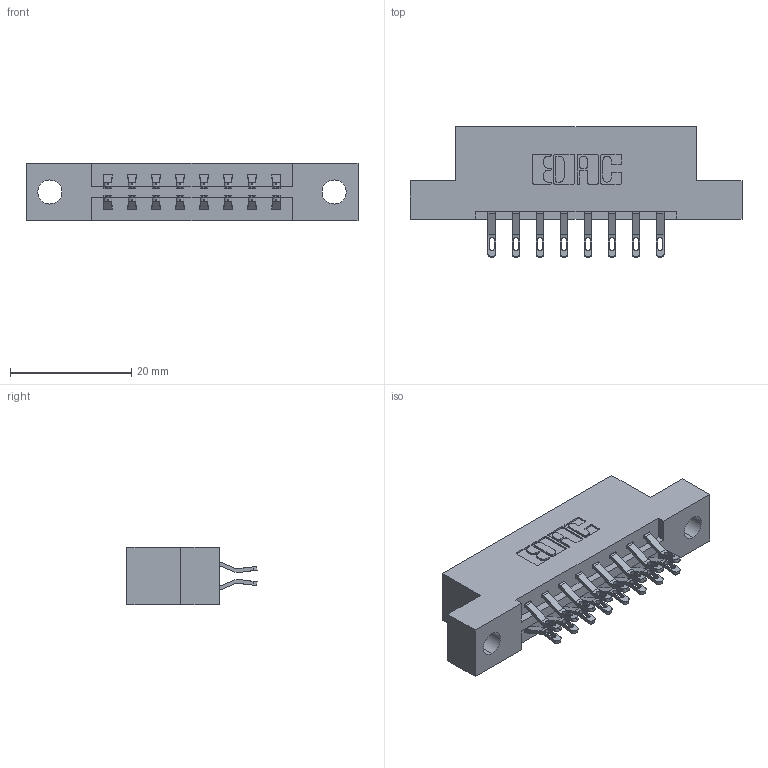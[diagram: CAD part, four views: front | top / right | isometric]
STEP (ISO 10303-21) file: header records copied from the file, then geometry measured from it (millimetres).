
FILE_DESCRIPTION (( 'STEP AP203' ), '1' );
FILE_NAME ('387-016-555-204.STEP', '2018-09-11T11:51:44', ( '' ), ( '' ), 'SwSTEP 2.0', 'SolidWorks 2016', '' );
FILE_SCHEMA (( 'CONFIG_CONTROL_DESIGN' ));
Length unit declared in the file: inch
Products named in the file (3): 387-016-555-204; 337 Part_Flush Mounting Lugs - 0.156 Dia-TH; 345-292-001_555 Tail
Assembly tree (17 placements, depth 2):
  387-016-555-204
    337 Part_Flush Mounting Lugs - 0.156 Dia-TH
    345-292-001_555 Tail  x16
Bounding box: 54.71 x 21.47 x 9.4 mm (x, y, z)
Volume: 5271.9 mm3; surface area: 5601.9 mm2
Topology: 17 solids, 17 shells, 1074 faces, 3335 edges, 2222 vertices
Faces by surface type: plane 646, cylinder 428
Entity records: 10929 total; most frequent: CARTESIAN_POINT 1904, ORIENTED_EDGE 1810, DIRECTION 1653, EDGE_CURVE 905, LINE 757, VECTOR 757, VERTEX_POINT 602, AXIS2_PLACEMENT_3D 448
